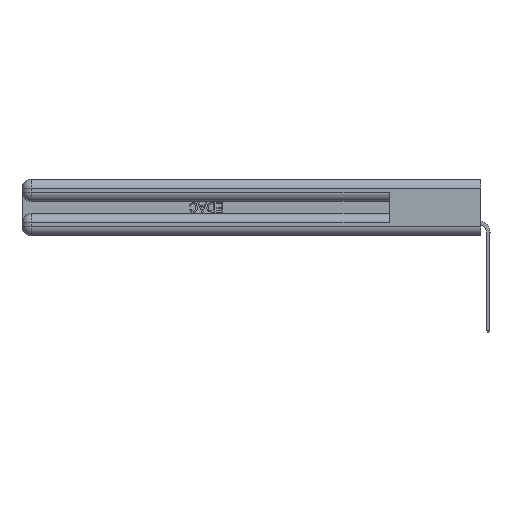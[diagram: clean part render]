
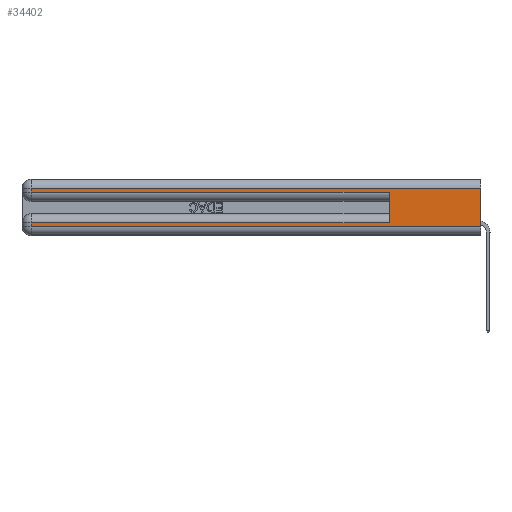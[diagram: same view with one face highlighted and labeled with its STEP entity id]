
A CAD part, left-side view. The second image highlights one B-rep face of the part: STEP entity #34402.
In plain terms, the highlighted planar face has unit normal (-1, 0, 0).
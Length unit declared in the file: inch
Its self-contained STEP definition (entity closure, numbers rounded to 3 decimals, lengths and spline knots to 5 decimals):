
#381 = VECTOR ( 'NONE', #12965, 39.37008 ) ;
#2254 = EDGE_CURVE ( 'NONE', #21955, #49012, #44126, .T. ) ;
#3604 = DIRECTION ( 'NONE',  ( 0., 0., 1. ) ) ;
#4623 = EDGE_CURVE ( 'NONE', #21955, #54637, #32510, .T. ) ;
#5341 = CARTESIAN_POINT ( 'NONE',  ( 0., 0., 0.085 ) ) ;
#5585 = VERTEX_POINT ( 'NONE', #24923 ) ;
#5713 = VECTOR ( 'NONE', #13323, 39.37008 ) ;
#5771 = CARTESIAN_POINT ( 'NONE',  ( 0., 0.6, 0.085 ) ) ;
#8515 = CARTESIAN_POINT ( 'NONE',  ( 0., 0., 0.31 ) ) ;
#8901 = ORIENTED_EDGE ( 'NONE', *, *, #45236, .T. ) ;
#10151 = ORIENTED_EDGE ( 'NONE', *, *, #14711, .T. ) ;
#12363 = EDGE_CURVE ( 'NONE', #17254, #25373, #44810, .T. ) ;
#12965 = DIRECTION ( 'NONE',  ( 0., 1., 0. ) ) ;
#13323 = DIRECTION ( 'NONE',  ( 0., 0., -1. ) ) ;
#14711 = EDGE_CURVE ( 'NONE', #31527, #5585, #37254, .T. ) ;
#15032 = ORIENTED_EDGE ( 'NONE', *, *, #4623, .F. ) ;
#15154 = VECTOR ( 'NONE', #19182, 39.37008 ) ;
#17254 = VERTEX_POINT ( 'NONE', #25090 ) ;
#17270 = DIRECTION ( 'NONE',  ( 1., 0., 0. ) ) ;
#17440 = PLANE ( 'NONE',  #30180 ) ;
#18777 = CARTESIAN_POINT ( 'NONE',  ( 0., 2.94, 0.285 ) ) ;
#18972 = ORIENTED_EDGE ( 'NONE', *, *, #26828, .F. ) ;
#19182 = DIRECTION ( 'NONE',  ( 0., -1., 0. ) ) ;
#20079 = VECTOR ( 'NONE', #26795, 39.37008 ) ;
#20628 = ORIENTED_EDGE ( 'NONE', *, *, #44007, .T. ) ;
#20973 = ORIENTED_EDGE ( 'NONE', *, *, #12363, .T. ) ;
#21955 = VERTEX_POINT ( 'NONE', #5771 ) ;
#21957 = FACE_OUTER_BOUND ( 'NONE', #24381, .T. ) ;
#22776 = VECTOR ( 'NONE', #36970, 39.37008 ) ;
#22900 = CARTESIAN_POINT ( 'NONE',  ( 0., 2.94, 0.37 ) ) ;
#24381 = EDGE_LOOP ( 'NONE', ( #18972, #10151, #8901, #52176, #15032, #38712, #20628, #20973 ) ) ;
#24417 = CARTESIAN_POINT ( 'NONE',  ( 0., 2.94, 0.085 ) ) ;
#24923 = CARTESIAN_POINT ( 'NONE',  ( 0., 2.94, 0.31 ) ) ;
#25090 = CARTESIAN_POINT ( 'NONE',  ( 0., 2.94, 0.06 ) ) ;
#25373 = VERTEX_POINT ( 'NONE', #44326 ) ;
#26795 = DIRECTION ( 'NONE',  ( 0., 1., 0. ) ) ;
#26828 = EDGE_CURVE ( 'NONE', #31527, #25373, #54986, .T. ) ;
#30180 = AXIS2_PLACEMENT_3D ( 'NONE', #47577, #17270, #38948 ) ;
#31527 = VERTEX_POINT ( 'NONE', #42401 ) ;
#32510 = LINE ( 'NONE', #33097, #51820 ) ;
#33097 = CARTESIAN_POINT ( 'NONE',  ( 0., 0.6, 0.145 ) ) ;
#33458 = VECTOR ( 'NONE', #51297, 39.37008 ) ;
#34402 = ADVANCED_FACE ( 'NONE', ( #21957 ), #17440, .F. ) ;
#34483 = CARTESIAN_POINT ( 'NONE',  ( 0., 2.94, 0.37 ) ) ;
#36510 = LINE ( 'NONE', #34483, #5713 ) ;
#36970 = DIRECTION ( 'NONE',  ( 0., 0., -1. ) ) ;
#37254 = LINE ( 'NONE', #8515, #381 ) ;
#38712 = ORIENTED_EDGE ( 'NONE', *, *, #2254, .T. ) ;
#38948 = DIRECTION ( 'NONE',  ( 0., 0., -1. ) ) ;
#39007 = EDGE_CURVE ( 'NONE', #40578, #54637, #43276, .T. ) ;
#40578 = VERTEX_POINT ( 'NONE', #18777 ) ;
#42401 = CARTESIAN_POINT ( 'NONE',  ( 0., 0., 0.31 ) ) ;
#42730 = CARTESIAN_POINT ( 'NONE',  ( 0., 0., 0.06 ) ) ;
#43276 = LINE ( 'NONE', #44245, #15154 ) ;
#44007 = EDGE_CURVE ( 'NONE', #49012, #17254, #45360, .T. ) ;
#44126 = LINE ( 'NONE', #5341, #20079 ) ;
#44245 = CARTESIAN_POINT ( 'NONE',  ( 0., 0., 0.285 ) ) ;
#44326 = CARTESIAN_POINT ( 'NONE',  ( 0., 0., 0.06 ) ) ;
#44625 = CARTESIAN_POINT ( 'NONE',  ( 0., 0.6, 0.285 ) ) ;
#44810 = LINE ( 'NONE', #42730, #33458 ) ;
#45236 = EDGE_CURVE ( 'NONE', #5585, #40578, #36510, .T. ) ;
#45360 = LINE ( 'NONE', #22900, #46097 ) ;
#46097 = VECTOR ( 'NONE', #53638, 39.37008 ) ;
#47577 = CARTESIAN_POINT ( 'NONE',  ( 0., 0., 0.37 ) ) ;
#49012 = VERTEX_POINT ( 'NONE', #24417 ) ;
#51069 = CARTESIAN_POINT ( 'NONE',  ( 0., 0., 0.37 ) ) ;
#51297 = DIRECTION ( 'NONE',  ( 0., -1., 0. ) ) ;
#51820 = VECTOR ( 'NONE', #3604, 39.37008 ) ;
#52176 = ORIENTED_EDGE ( 'NONE', *, *, #39007, .T. ) ;
#53638 = DIRECTION ( 'NONE',  ( 0., 0., -1. ) ) ;
#54637 = VERTEX_POINT ( 'NONE', #44625 ) ;
#54986 = LINE ( 'NONE', #51069, #22776 ) ;
